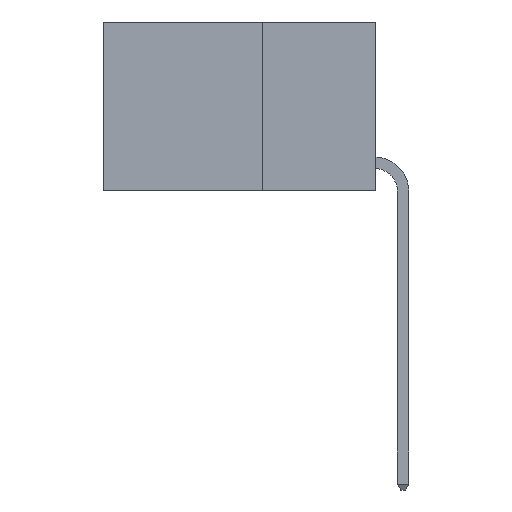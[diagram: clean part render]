
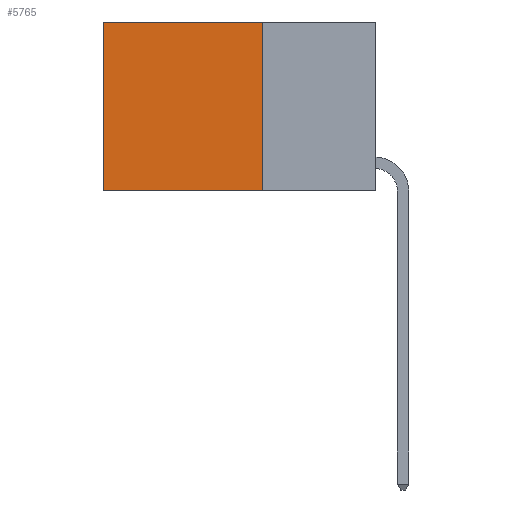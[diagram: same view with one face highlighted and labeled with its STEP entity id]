
A CAD part, left-side view. The second image highlights one B-rep face of the part: STEP entity #5765.
In plain terms, the highlighted planar face has unit normal (-1, 0, 0).
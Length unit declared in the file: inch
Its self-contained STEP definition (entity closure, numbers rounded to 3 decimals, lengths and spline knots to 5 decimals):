
#561 = CARTESIAN_POINT ( 'NONE',  ( 0.2625, 0.6, 0. ) ) ;
#665 = VECTOR ( 'NONE', #7463, 39.37008 ) ;
#1044 = EDGE_CURVE ( 'NONE', #1813, #2802, #5972, .T. ) ;
#1166 = CARTESIAN_POINT ( 'NONE',  ( 0.2625, 0.25, 0. ) ) ;
#1813 = VERTEX_POINT ( 'NONE', #4295 ) ;
#1974 = DIRECTION ( 'NONE',  ( 1., 0., 0. ) ) ;
#2283 = EDGE_CURVE ( 'NONE', #8421, #8645, #8848, .T. ) ;
#2328 = DIRECTION ( 'NONE',  ( 0., 0., -1. ) ) ;
#2802 = VERTEX_POINT ( 'NONE', #561 ) ;
#3009 = AXIS2_PLACEMENT_3D ( 'NONE', #1166, #1974, #7464 ) ;
#3025 = FACE_OUTER_BOUND ( 'NONE', #3928, .T. ) ;
#3377 = ORIENTED_EDGE ( 'NONE', *, *, #8732, .T. ) ;
#3928 = EDGE_LOOP ( 'NONE', ( #3377, #4163, #8635, #8088 ) ) ;
#4163 = ORIENTED_EDGE ( 'NONE', *, *, #2283, .F. ) ;
#4295 = CARTESIAN_POINT ( 'NONE',  ( 0.2625, 0.25, 0. ) ) ;
#4951 = LINE ( 'NONE', #9804, #665 ) ;
#5079 = CARTESIAN_POINT ( 'NONE',  ( 0.2625, 0.6, -0.37 ) ) ;
#5471 = CARTESIAN_POINT ( 'NONE',  ( 0.2625, 0.25, -0.37 ) ) ;
#5472 = CARTESIAN_POINT ( 'NONE',  ( 0.2625, 0.25, 0. ) ) ;
#5493 = EDGE_CURVE ( 'NONE', #1813, #8421, #6281, .T. ) ;
#5765 = ADVANCED_FACE ( 'NONE', ( #3025 ), #5908, .F. ) ;
#5908 = PLANE ( 'NONE',  #3009 ) ;
#5972 = LINE ( 'NONE', #8365, #6126 ) ;
#6126 = VECTOR ( 'NONE', #8710, 39.37008 ) ;
#6281 = LINE ( 'NONE', #5472, #7147 ) ;
#6297 = CARTESIAN_POINT ( 'NONE',  ( 0.2625, 0.25, -0.37 ) ) ;
#7147 = VECTOR ( 'NONE', #2328, 39.37008 ) ;
#7463 = DIRECTION ( 'NONE',  ( 0., 0., -1. ) ) ;
#7464 = DIRECTION ( 'NONE',  ( 0., 0., -1. ) ) ;
#8088 = ORIENTED_EDGE ( 'NONE', *, *, #1044, .T. ) ;
#8365 = CARTESIAN_POINT ( 'NONE',  ( 0.2625, 0.25, 0. ) ) ;
#8421 = VERTEX_POINT ( 'NONE', #5471 ) ;
#8635 = ORIENTED_EDGE ( 'NONE', *, *, #5493, .F. ) ;
#8645 = VERTEX_POINT ( 'NONE', #5079 ) ;
#8697 = DIRECTION ( 'NONE',  ( 0., 1., 0. ) ) ;
#8710 = DIRECTION ( 'NONE',  ( 0., 1., 0. ) ) ;
#8732 = EDGE_CURVE ( 'NONE', #2802, #8645, #4951, .T. ) ;
#8758 = VECTOR ( 'NONE', #8697, 39.37008 ) ;
#8848 = LINE ( 'NONE', #6297, #8758 ) ;
#9804 = CARTESIAN_POINT ( 'NONE',  ( 0.2625, 0.6, 0. ) ) ;
